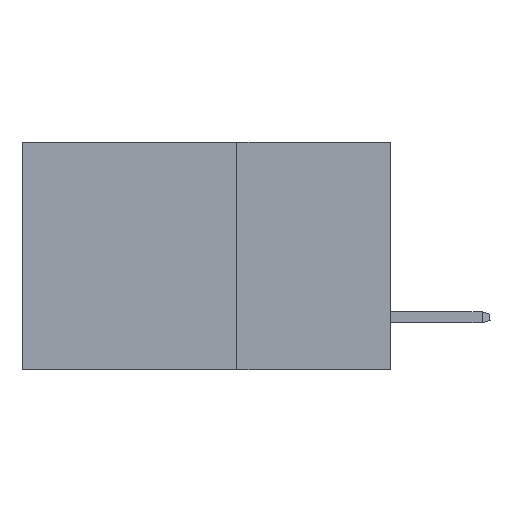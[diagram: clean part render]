
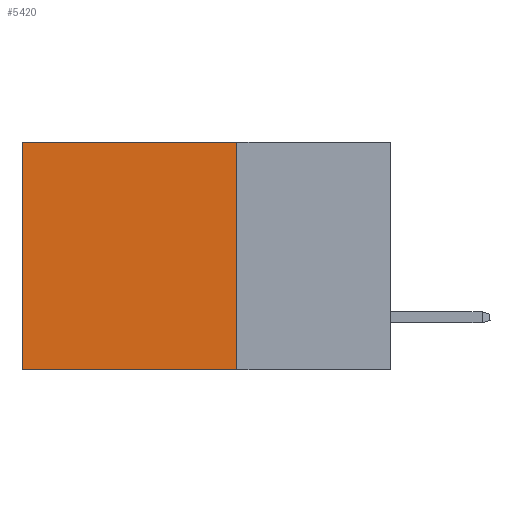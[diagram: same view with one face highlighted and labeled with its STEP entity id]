
A CAD part, left-side view. The second image highlights one B-rep face of the part: STEP entity #5420.
In plain terms, the highlighted planar face has unit normal (-1, 0, 0).
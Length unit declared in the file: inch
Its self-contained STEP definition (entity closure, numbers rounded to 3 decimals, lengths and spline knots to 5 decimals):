
#437 = EDGE_LOOP ( 'NONE', ( #4557, #6379, #9246, #4272 ) ) ;
#444 = CARTESIAN_POINT ( 'NONE',  ( 0.2875, 0.6, 0. ) ) ;
#587 = VERTEX_POINT ( 'NONE', #7458 ) ;
#937 = LINE ( 'NONE', #3983, #5630 ) ;
#960 = CARTESIAN_POINT ( 'NONE',  ( 0.2875, 0.25, 0. ) ) ;
#1140 = DIRECTION ( 'NONE',  ( 0., 0., -1. ) ) ;
#1725 = LINE ( 'NONE', #6884, #2671 ) ;
#2113 = DIRECTION ( 'NONE',  ( 1., 0., 0. ) ) ;
#2145 = PLANE ( 'NONE',  #4552 ) ;
#2199 = LINE ( 'NONE', #4099, #5591 ) ;
#2671 = VECTOR ( 'NONE', #3454, 39.37008 ) ;
#3229 = EDGE_CURVE ( 'NONE', #3783, #4825, #8262, .T. ) ;
#3362 = DIRECTION ( 'NONE',  ( 0., 0., -1. ) ) ;
#3454 = DIRECTION ( 'NONE',  ( 0., 1., 0. ) ) ;
#3783 = VERTEX_POINT ( 'NONE', #7935 ) ;
#3983 = CARTESIAN_POINT ( 'NONE',  ( 0.2875, 0.6, 0. ) ) ;
#4099 = CARTESIAN_POINT ( 'NONE',  ( 0.2875, 0.25, 0. ) ) ;
#4272 = ORIENTED_EDGE ( 'NONE', *, *, #3229, .T. ) ;
#4552 = AXIS2_PLACEMENT_3D ( 'NONE', #7227, #2113, #9359 ) ;
#4557 = ORIENTED_EDGE ( 'NONE', *, *, #6275, .T. ) ;
#4641 = VERTEX_POINT ( 'NONE', #5528 ) ;
#4825 = VERTEX_POINT ( 'NONE', #444 ) ;
#5420 = ADVANCED_FACE ( 'NONE', ( #7890 ), #2145, .F. ) ;
#5528 = CARTESIAN_POINT ( 'NONE',  ( 0.2875, 0.6, -0.37 ) ) ;
#5591 = VECTOR ( 'NONE', #3362, 39.37008 ) ;
#5630 = VECTOR ( 'NONE', #1140, 39.37008 ) ;
#5768 = EDGE_CURVE ( 'NONE', #3783, #587, #2199, .T. ) ;
#6275 = EDGE_CURVE ( 'NONE', #4825, #4641, #937, .T. ) ;
#6379 = ORIENTED_EDGE ( 'NONE', *, *, #7117, .F. ) ;
#6852 = DIRECTION ( 'NONE',  ( 0., 1., 0. ) ) ;
#6884 = CARTESIAN_POINT ( 'NONE',  ( 0.2875, 0.25, -0.37 ) ) ;
#7117 = EDGE_CURVE ( 'NONE', #587, #4641, #1725, .T. ) ;
#7227 = CARTESIAN_POINT ( 'NONE',  ( 0.2875, 0.25, 0. ) ) ;
#7458 = CARTESIAN_POINT ( 'NONE',  ( 0.2875, 0.25, -0.37 ) ) ;
#7890 = FACE_OUTER_BOUND ( 'NONE', #437, .T. ) ;
#7935 = CARTESIAN_POINT ( 'NONE',  ( 0.2875, 0.25, 0. ) ) ;
#8262 = LINE ( 'NONE', #960, #9055 ) ;
#9055 = VECTOR ( 'NONE', #6852, 39.37008 ) ;
#9246 = ORIENTED_EDGE ( 'NONE', *, *, #5768, .F. ) ;
#9359 = DIRECTION ( 'NONE',  ( 0., 0., -1. ) ) ;
